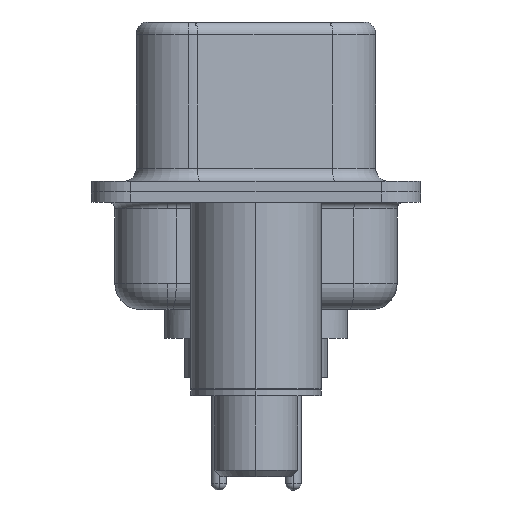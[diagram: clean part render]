
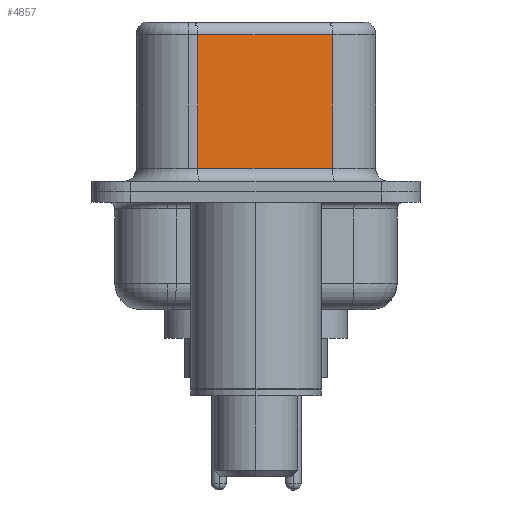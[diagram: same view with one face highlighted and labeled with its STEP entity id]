
A CAD part, left-side view. The second image highlights one B-rep face of the part: STEP entity #4857.
In plain terms, the highlighted planar face has unit normal (-0.985, -0.174, 0).
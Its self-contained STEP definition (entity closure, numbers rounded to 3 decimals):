
#602 = CARTESIAN_POINT ( 'NONE',  ( 3.67, 2.233, 0.9 ) ) ;
#2014 = EDGE_CURVE ( 'NONE', #6581, #11014, #14528, .T. ) ;
#2037 = DIRECTION ( 'NONE',  ( -0.174, 0.985, 0. ) ) ;
#2489 = ORIENTED_EDGE ( 'NONE', *, *, #14784, .F. ) ;
#2592 = LINE ( 'NONE', #8222, #20133 ) ;
#3150 = VERTEX_POINT ( 'NONE', #11253 ) ;
#3584 = VERTEX_POINT ( 'NONE', #17933 ) ;
#4438 = AXIS2_PLACEMENT_3D ( 'NONE', #13002, #6207, #2037 ) ;
#4857 = ADVANCED_FACE ( 'NONE', ( #19210 ), #7071, .F. ) ;
#6207 = DIRECTION ( 'NONE',  ( 0.985, 0.174, 0. ) ) ;
#6384 = VECTOR ( 'NONE', #9767, 1000. ) ;
#6581 = VERTEX_POINT ( 'NONE', #10483 ) ;
#7071 = PLANE ( 'NONE',  #4438 ) ;
#8222 = CARTESIAN_POINT ( 'NONE',  ( 4.58, -2.927, 6.02 ) ) ;
#8255 = DIRECTION ( 'NONE',  ( 0., 0., -1. ) ) ;
#8609 = CARTESIAN_POINT ( 'NONE',  ( 3.67, 2.233, 6.52 ) ) ;
#9767 = DIRECTION ( 'NONE',  ( 0.174, -0.985, 0. ) ) ;
#10027 = VECTOR ( 'NONE', #15591, 1000. ) ;
#10483 = CARTESIAN_POINT ( 'NONE',  ( 3.67, 2.233, 6.02 ) ) ;
#10893 = LINE ( 'NONE', #21516, #6384 ) ;
#11014 = VERTEX_POINT ( 'NONE', #602 ) ;
#11048 = LINE ( 'NONE', #16730, #19005 ) ;
#11089 = ORIENTED_EDGE ( 'NONE', *, *, #21202, .T. ) ;
#11253 = CARTESIAN_POINT ( 'NONE',  ( 4.58, -2.927, 0.9 ) ) ;
#11816 = EDGE_CURVE ( 'NONE', #11014, #3150, #10893, .T. ) ;
#13002 = CARTESIAN_POINT ( 'NONE',  ( 4.58, -2.927, 6.52 ) ) ;
#13255 = DIRECTION ( 'NONE',  ( -0.174, 0.985, 0. ) ) ;
#13331 = ORIENTED_EDGE ( 'NONE', *, *, #2014, .T. ) ;
#14528 = LINE ( 'NONE', #8609, #10027 ) ;
#14784 = EDGE_CURVE ( 'NONE', #3584, #3150, #11048, .T. ) ;
#15591 = DIRECTION ( 'NONE',  ( 0., 0., -1. ) ) ;
#16121 = EDGE_LOOP ( 'NONE', ( #2489, #11089, #13331, #17404 ) ) ;
#16730 = CARTESIAN_POINT ( 'NONE',  ( 4.58, -2.927, 6.52 ) ) ;
#17404 = ORIENTED_EDGE ( 'NONE', *, *, #11816, .T. ) ;
#17933 = CARTESIAN_POINT ( 'NONE',  ( 4.58, -2.927, 6.02 ) ) ;
#19005 = VECTOR ( 'NONE', #8255, 1000. ) ;
#19210 = FACE_OUTER_BOUND ( 'NONE', #16121, .T. ) ;
#20133 = VECTOR ( 'NONE', #13255, 1000. ) ;
#21202 = EDGE_CURVE ( 'NONE', #3584, #6581, #2592, .T. ) ;
#21516 = CARTESIAN_POINT ( 'NONE',  ( 4.58, -2.927, 0.9 ) ) ;
